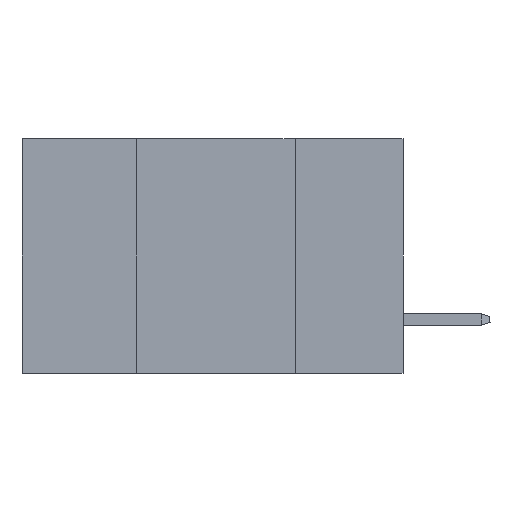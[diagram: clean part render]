
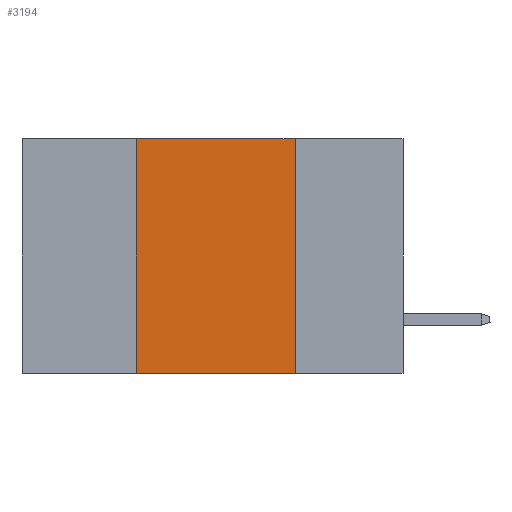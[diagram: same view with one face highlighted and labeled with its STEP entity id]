
A CAD part, left-side view. The second image highlights one B-rep face of the part: STEP entity #3194.
In plain terms, the highlighted planar face has unit normal (-1, 0, 0).
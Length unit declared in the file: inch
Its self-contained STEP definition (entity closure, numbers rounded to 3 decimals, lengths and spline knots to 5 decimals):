
#395 = CARTESIAN_POINT ( 'NONE',  ( 0., 0.17, 0. ) ) ;
#989 = AXIS2_PLACEMENT_3D ( 'NONE', #10891, #18393, #18685 ) ;
#1671 = CARTESIAN_POINT ( 'NONE',  ( 0., 0.6, 0. ) ) ;
#2708 = VECTOR ( 'NONE', #18579, 39.37008 ) ;
#3194 = ADVANCED_FACE ( 'NONE', ( #12207 ), #9368, .F. ) ;
#3894 = EDGE_CURVE ( 'NONE', #18361, #14727, #19480, .T. ) ;
#5300 = EDGE_CURVE ( 'NONE', #9388, #14727, #16464, .T. ) ;
#5349 = ORIENTED_EDGE ( 'NONE', *, *, #8150, .F. ) ;
#5473 = DIRECTION ( 'NONE',  ( 0., -1., 0. ) ) ;
#5490 = EDGE_LOOP ( 'NONE', ( #9489, #5349, #12327, #6155 ) ) ;
#5669 = CARTESIAN_POINT ( 'NONE',  ( 0., 0.6, -0.37 ) ) ;
#5854 = CARTESIAN_POINT ( 'NONE',  ( 0., 0.42, 0. ) ) ;
#6108 = CARTESIAN_POINT ( 'NONE',  ( 0., 0.42, 0. ) ) ;
#6155 = ORIENTED_EDGE ( 'NONE', *, *, #3894, .T. ) ;
#6265 = VERTEX_POINT ( 'NONE', #5854 ) ;
#7031 = DIRECTION ( 'NONE',  ( 0., 0., -1. ) ) ;
#7733 = LINE ( 'NONE', #6108, #2708 ) ;
#8069 = LINE ( 'NONE', #1671, #16884 ) ;
#8150 = EDGE_CURVE ( 'NONE', #6265, #9388, #8069, .T. ) ;
#9368 = PLANE ( 'NONE',  #989 ) ;
#9388 = VERTEX_POINT ( 'NONE', #395 ) ;
#9489 = ORIENTED_EDGE ( 'NONE', *, *, #5300, .F. ) ;
#9949 = VECTOR ( 'NONE', #5473, 39.37008 ) ;
#10322 = VECTOR ( 'NONE', #7031, 39.37008 ) ;
#10891 = CARTESIAN_POINT ( 'NONE',  ( 0., 0.6, 0. ) ) ;
#12207 = FACE_OUTER_BOUND ( 'NONE', #5490, .T. ) ;
#12327 = ORIENTED_EDGE ( 'NONE', *, *, #12991, .F. ) ;
#12991 = EDGE_CURVE ( 'NONE', #18361, #6265, #7733, .T. ) ;
#14054 = CARTESIAN_POINT ( 'NONE',  ( 0., 0.42, -0.37 ) ) ;
#14727 = VERTEX_POINT ( 'NONE', #15428 ) ;
#15428 = CARTESIAN_POINT ( 'NONE',  ( 0., 0.17, -0.37 ) ) ;
#16464 = LINE ( 'NONE', #19300, #10322 ) ;
#16884 = VECTOR ( 'NONE', #17209, 39.37008 ) ;
#17209 = DIRECTION ( 'NONE',  ( 0., -1., 0. ) ) ;
#18361 = VERTEX_POINT ( 'NONE', #14054 ) ;
#18393 = DIRECTION ( 'NONE',  ( 1., 0., 0. ) ) ;
#18579 = DIRECTION ( 'NONE',  ( 0., 0., 1. ) ) ;
#18685 = DIRECTION ( 'NONE',  ( 0., 0., -1. ) ) ;
#19300 = CARTESIAN_POINT ( 'NONE',  ( 0., 0.17, 0. ) ) ;
#19480 = LINE ( 'NONE', #5669, #9949 ) ;
